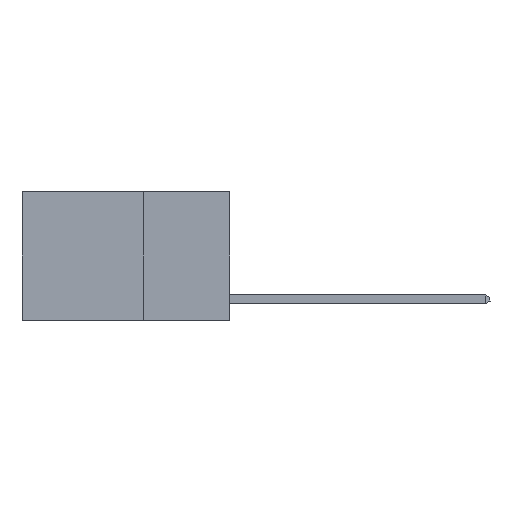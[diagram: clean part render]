
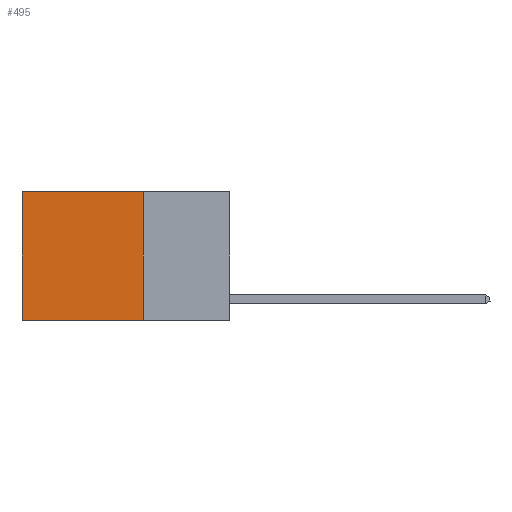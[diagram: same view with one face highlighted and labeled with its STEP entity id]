
A CAD part, left-side view. The second image highlights one B-rep face of the part: STEP entity #495.
In plain terms, the highlighted planar face has unit normal (-1, 0, 0).
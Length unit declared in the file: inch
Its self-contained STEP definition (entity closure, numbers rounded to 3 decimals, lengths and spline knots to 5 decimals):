
#495 = ADVANCED_FACE ( 'NONE', ( #2316 ), #29718, .F. ) ;
#525 = EDGE_CURVE ( 'NONE', #17512, #16390, #846, .T. ) ;
#846 = LINE ( 'NONE', #10861, #26778 ) ;
#1334 = DIRECTION ( 'NONE',  ( 1., 0., 0. ) ) ;
#2316 = FACE_OUTER_BOUND ( 'NONE', #19832, .T. ) ;
#3809 = ORIENTED_EDGE ( 'NONE', *, *, #525, .T. ) ;
#5491 = DIRECTION ( 'NONE',  ( 0., 0., -1. ) ) ;
#6629 = VECTOR ( 'NONE', #14960, 39.37008 ) ;
#8120 = LINE ( 'NONE', #10192, #6629 ) ;
#9037 = VECTOR ( 'NONE', #21242, 39.37008 ) ;
#9405 = CARTESIAN_POINT ( 'NONE',  ( 0.2625, 0.25, -0.37 ) ) ;
#9765 = LINE ( 'NONE', #9405, #9037 ) ;
#9994 = CARTESIAN_POINT ( 'NONE',  ( 0.2625, 0.6, -0.37 ) ) ;
#10192 = CARTESIAN_POINT ( 'NONE',  ( 0.2625, 0.25, 0. ) ) ;
#10861 = CARTESIAN_POINT ( 'NONE',  ( 0.2625, 0.6, 0. ) ) ;
#12614 = CARTESIAN_POINT ( 'NONE',  ( 0.2625, 0.6, 0. ) ) ;
#13244 = DIRECTION ( 'NONE',  ( 0., 0., -1. ) ) ;
#14278 = VECTOR ( 'NONE', #5491, 39.37008 ) ;
#14960 = DIRECTION ( 'NONE',  ( 0., 1., 0. ) ) ;
#15519 = CARTESIAN_POINT ( 'NONE',  ( 0.2625, 0.25, 0. ) ) ;
#16390 = VERTEX_POINT ( 'NONE', #9994 ) ;
#17371 = VERTEX_POINT ( 'NONE', #23925 ) ;
#17512 = VERTEX_POINT ( 'NONE', #12614 ) ;
#17918 = DIRECTION ( 'NONE',  ( 0., 0., -1. ) ) ;
#19832 = EDGE_LOOP ( 'NONE', ( #3809, #19950, #27759, #21379 ) ) ;
#19950 = ORIENTED_EDGE ( 'NONE', *, *, #23564, .F. ) ;
#20135 = EDGE_CURVE ( 'NONE', #30491, #17512, #8120, .T. ) ;
#20338 = AXIS2_PLACEMENT_3D ( 'NONE', #15519, #1334, #17918 ) ;
#20601 = LINE ( 'NONE', #22075, #14278 ) ;
#21242 = DIRECTION ( 'NONE',  ( 0., 1., 0. ) ) ;
#21379 = ORIENTED_EDGE ( 'NONE', *, *, #20135, .T. ) ;
#22075 = CARTESIAN_POINT ( 'NONE',  ( 0.2625, 0.25, 0. ) ) ;
#23564 = EDGE_CURVE ( 'NONE', #17371, #16390, #9765, .T. ) ;
#23925 = CARTESIAN_POINT ( 'NONE',  ( 0.2625, 0.25, -0.37 ) ) ;
#26778 = VECTOR ( 'NONE', #13244, 39.37008 ) ;
#27759 = ORIENTED_EDGE ( 'NONE', *, *, #28131, .F. ) ;
#28131 = EDGE_CURVE ( 'NONE', #30491, #17371, #20601, .T. ) ;
#29718 = PLANE ( 'NONE',  #20338 ) ;
#30491 = VERTEX_POINT ( 'NONE', #30634 ) ;
#30634 = CARTESIAN_POINT ( 'NONE',  ( 0.2625, 0.25, 0. ) ) ;
